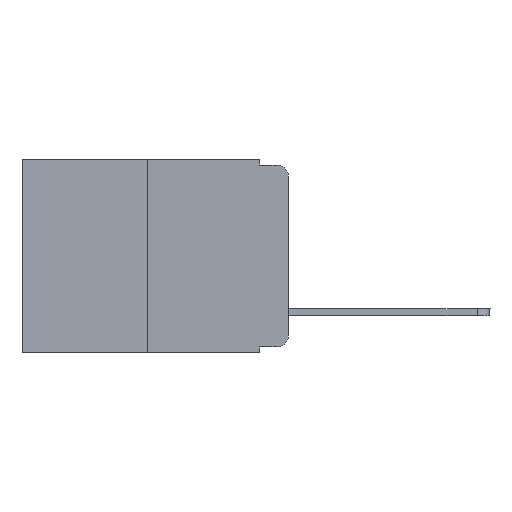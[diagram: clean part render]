
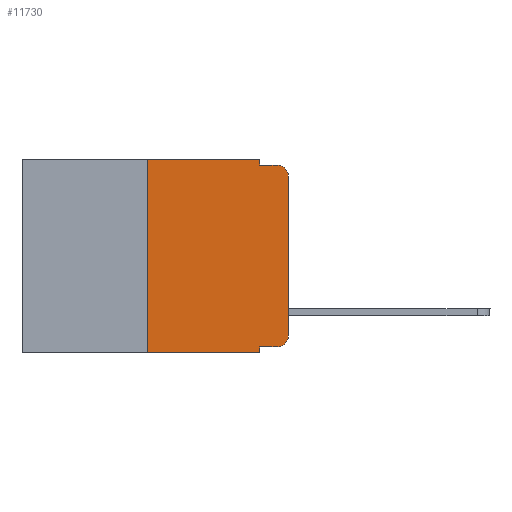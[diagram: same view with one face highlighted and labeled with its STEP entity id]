
A CAD part, left-side view. The second image highlights one B-rep face of the part: STEP entity #11730.
In plain terms, the highlighted planar face has unit normal (-1, 0, 0).
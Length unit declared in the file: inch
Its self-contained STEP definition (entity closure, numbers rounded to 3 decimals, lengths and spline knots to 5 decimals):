
#38 = EDGE_CURVE ( 'NONE', #2070, #17723, #14508, .T. ) ;
#201 = CARTESIAN_POINT ( 'NONE',  ( 0., 0.051, -0.333 ) ) ;
#851 = CARTESIAN_POINT ( 'NONE',  ( 0., 0.02, -0.01 ) ) ;
#921 = DIRECTION ( 'NONE',  ( 0., -1., 0. ) ) ;
#1039 = LINE ( 'NONE', #22649, #16580 ) ;
#1729 = ORIENTED_EDGE ( 'NONE', *, *, #11594, .F. ) ;
#2070 = VERTEX_POINT ( 'NONE', #18291 ) ;
#2243 = EDGE_LOOP ( 'NONE', ( #2757, #16064, #8380, #1729, #14014, #3198, #9680, #3799, #20168, #17958 ) ) ;
#2373 = VECTOR ( 'NONE', #7459, 39.37008 ) ;
#2659 = DIRECTION ( 'NONE',  ( 0., 0., 1. ) ) ;
#2757 = ORIENTED_EDGE ( 'NONE', *, *, #3967, .T. ) ;
#2788 = CARTESIAN_POINT ( 'NONE',  ( 0., 0.473, 0. ) ) ;
#2997 = DIRECTION ( 'NONE',  ( -1., 0., 0. ) ) ;
#3198 = ORIENTED_EDGE ( 'NONE', *, *, #11656, .F. ) ;
#3345 = VERTEX_POINT ( 'NONE', #19727 ) ;
#3618 = CARTESIAN_POINT ( 'NONE',  ( 0., 0.051, 0. ) ) ;
#3737 = CARTESIAN_POINT ( 'NONE',  ( 0., 0.051, -0.01 ) ) ;
#3799 = ORIENTED_EDGE ( 'NONE', *, *, #21271, .F. ) ;
#3839 = EDGE_CURVE ( 'NONE', #3345, #18375, #7118, .T. ) ;
#3967 = EDGE_CURVE ( 'NONE', #4919, #13169, #20149, .T. ) ;
#4311 = DIRECTION ( 'NONE',  ( 0., 0., 1. ) ) ;
#4323 = CARTESIAN_POINT ( 'NONE',  ( 0., 0.02, -0.03 ) ) ;
#4919 = VERTEX_POINT ( 'NONE', #5920 ) ;
#5320 = CARTESIAN_POINT ( 'NONE',  ( 0., 0.051, 0. ) ) ;
#5735 = DIRECTION ( 'NONE',  ( 0., -1., 0. ) ) ;
#5920 = CARTESIAN_POINT ( 'NONE',  ( 0., 0., -0.313 ) ) ;
#6503 = CIRCLE ( 'NONE', #13623, 0.02 ) ;
#7118 = LINE ( 'NONE', #201, #2373 ) ;
#7459 = DIRECTION ( 'NONE',  ( 0., -1., 0. ) ) ;
#8071 = CARTESIAN_POINT ( 'NONE',  ( 0., 0.051, -0.01 ) ) ;
#8177 = FACE_OUTER_BOUND ( 'NONE', #2243, .T. ) ;
#8380 = ORIENTED_EDGE ( 'NONE', *, *, #20213, .F. ) ;
#8532 = CARTESIAN_POINT ( 'NONE',  ( 0., 0., -0.03 ) ) ;
#8661 = VECTOR ( 'NONE', #4311, 39.37008 ) ;
#9043 = AXIS2_PLACEMENT_3D ( 'NONE', #2788, #15347, #9829 ) ;
#9632 = VERTEX_POINT ( 'NONE', #851 ) ;
#9680 = ORIENTED_EDGE ( 'NONE', *, *, #38, .T. ) ;
#9829 = DIRECTION ( 'NONE',  ( 0., 0., -1. ) ) ;
#9834 = CARTESIAN_POINT ( 'NONE',  ( 0., 0.473, 0. ) ) ;
#9842 = DIRECTION ( 'NONE',  ( 0., 0., -1. ) ) ;
#9919 = CARTESIAN_POINT ( 'NONE',  ( 0., 0.473, -0.343 ) ) ;
#11594 = EDGE_CURVE ( 'NONE', #21769, #12945, #18289, .T. ) ;
#11656 = EDGE_CURVE ( 'NONE', #2070, #19377, #18992, .T. ) ;
#11730 = ADVANCED_FACE ( 'NONE', ( #8177 ), #13579, .F. ) ;
#11847 = VECTOR ( 'NONE', #15442, 39.37008 ) ;
#11911 = CARTESIAN_POINT ( 'NONE',  ( 0., 0.02, -0.313 ) ) ;
#12144 = DIRECTION ( 'NONE',  ( 0., 0., -1. ) ) ;
#12945 = VERTEX_POINT ( 'NONE', #8071 ) ;
#13169 = VERTEX_POINT ( 'NONE', #8532 ) ;
#13535 = VECTOR ( 'NONE', #16535, 39.37008 ) ;
#13579 = PLANE ( 'NONE',  #9043 ) ;
#13623 = AXIS2_PLACEMENT_3D ( 'NONE', #4323, #22059, #9842 ) ;
#13800 = CARTESIAN_POINT ( 'NONE',  ( 0., 0.051, -0.343 ) ) ;
#13917 = VECTOR ( 'NONE', #921, 39.37008 ) ;
#14014 = ORIENTED_EDGE ( 'NONE', *, *, #20374, .F. ) ;
#14508 = LINE ( 'NONE', #9919, #11847 ) ;
#15245 = DIRECTION ( 'NONE',  ( 0., 0., -1. ) ) ;
#15328 = CARTESIAN_POINT ( 'NONE',  ( 0., 0., 0. ) ) ;
#15347 = DIRECTION ( 'NONE',  ( 1., 0., 0. ) ) ;
#15442 = DIRECTION ( 'NONE',  ( 0., -1., 0. ) ) ;
#16064 = ORIENTED_EDGE ( 'NONE', *, *, #22356, .T. ) ;
#16308 = LINE ( 'NONE', #3737, #19922 ) ;
#16535 = DIRECTION ( 'NONE',  ( 0., 0., -1. ) ) ;
#16580 = VECTOR ( 'NONE', #15245, 39.37008 ) ;
#16778 = LINE ( 'NONE', #9834, #13917 ) ;
#16877 = CIRCLE ( 'NONE', #17996, 0.02 ) ;
#17032 = EDGE_CURVE ( 'NONE', #18375, #4919, #16877, .T. ) ;
#17723 = VERTEX_POINT ( 'NONE', #13800 ) ;
#17958 = ORIENTED_EDGE ( 'NONE', *, *, #17032, .T. ) ;
#17996 = AXIS2_PLACEMENT_3D ( 'NONE', #11911, #2997, #12144 ) ;
#18289 = LINE ( 'NONE', #3618, #13535 ) ;
#18291 = CARTESIAN_POINT ( 'NONE',  ( 0., 0.25, -0.343 ) ) ;
#18375 = VERTEX_POINT ( 'NONE', #22109 ) ;
#18530 = CARTESIAN_POINT ( 'NONE',  ( 0., 0.25, 0. ) ) ;
#18992 = LINE ( 'NONE', #18530, #8661 ) ;
#19377 = VERTEX_POINT ( 'NONE', #22834 ) ;
#19727 = CARTESIAN_POINT ( 'NONE',  ( 0., 0.051, -0.333 ) ) ;
#19922 = VECTOR ( 'NONE', #5735, 39.37008 ) ;
#20149 = LINE ( 'NONE', #15328, #23171 ) ;
#20168 = ORIENTED_EDGE ( 'NONE', *, *, #3839, .T. ) ;
#20213 = EDGE_CURVE ( 'NONE', #12945, #9632, #16308, .T. ) ;
#20374 = EDGE_CURVE ( 'NONE', #19377, #21769, #16778, .T. ) ;
#21271 = EDGE_CURVE ( 'NONE', #3345, #17723, #1039, .T. ) ;
#21769 = VERTEX_POINT ( 'NONE', #5320 ) ;
#22059 = DIRECTION ( 'NONE',  ( -1., 0., 0. ) ) ;
#22109 = CARTESIAN_POINT ( 'NONE',  ( 0., 0.02, -0.333 ) ) ;
#22356 = EDGE_CURVE ( 'NONE', #13169, #9632, #6503, .T. ) ;
#22649 = CARTESIAN_POINT ( 'NONE',  ( 0., 0.051, 0. ) ) ;
#22834 = CARTESIAN_POINT ( 'NONE',  ( 0., 0.25, 0. ) ) ;
#23171 = VECTOR ( 'NONE', #2659, 39.37008 ) ;
